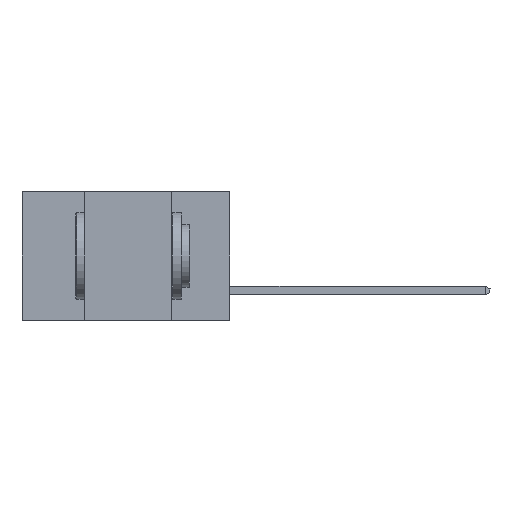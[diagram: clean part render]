
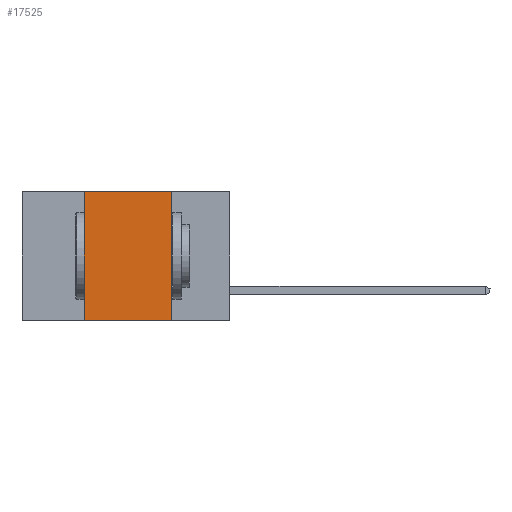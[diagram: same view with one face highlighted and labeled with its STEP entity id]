
A CAD part, left-side view. The second image highlights one B-rep face of the part: STEP entity #17525.
In plain terms, the highlighted planar face has unit normal (-1, 0, 0).
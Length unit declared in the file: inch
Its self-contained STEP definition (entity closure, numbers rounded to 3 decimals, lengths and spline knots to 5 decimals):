
#531 = AXIS2_PLACEMENT_3D ( 'NONE', #15701, #7742, #21314 ) ;
#1015 = EDGE_CURVE ( 'NONE', #6487, #20729, #23118, .T. ) ;
#1554 = CARTESIAN_POINT ( 'NONE',  ( 0., 0.17, -0.37 ) ) ;
#3136 = DIRECTION ( 'NONE',  ( 0., 0., -1. ) ) ;
#3268 = LINE ( 'NONE', #11237, #25562 ) ;
#4190 = LINE ( 'NONE', #19735, #8039 ) ;
#6487 = VERTEX_POINT ( 'NONE', #13993 ) ;
#6577 = EDGE_CURVE ( 'NONE', #20702, #20729, #4190, .T. ) ;
#6822 = EDGE_CURVE ( 'NONE', #20702, #9094, #3268, .T. ) ;
#7489 = FACE_OUTER_BOUND ( 'NONE', #17699, .T. ) ;
#7742 = DIRECTION ( 'NONE',  ( 1., 0., 0. ) ) ;
#8039 = VECTOR ( 'NONE', #10194, 39.37008 ) ;
#9094 = VERTEX_POINT ( 'NONE', #25158 ) ;
#10194 = DIRECTION ( 'NONE',  ( 0., -1., 0. ) ) ;
#11237 = CARTESIAN_POINT ( 'NONE',  ( 0., 0.42, -0.37 ) ) ;
#11472 = ORIENTED_EDGE ( 'NONE', *, *, #1015, .F. ) ;
#13035 = CARTESIAN_POINT ( 'NONE',  ( 0., 0.6, 0. ) ) ;
#13333 = PLANE ( 'NONE',  #531 ) ;
#13993 = CARTESIAN_POINT ( 'NONE',  ( 0., 0.17, 0. ) ) ;
#14577 = VECTOR ( 'NONE', #3136, 39.37008 ) ;
#14610 = ORIENTED_EDGE ( 'NONE', *, *, #6577, .T. ) ;
#15701 = CARTESIAN_POINT ( 'NONE',  ( 0., 0.6, 0. ) ) ;
#16845 = DIRECTION ( 'NONE',  ( 0., -1., 0. ) ) ;
#17107 = LINE ( 'NONE', #13035, #24840 ) ;
#17124 = DIRECTION ( 'NONE',  ( 0., 0., 1. ) ) ;
#17525 = ADVANCED_FACE ( 'NONE', ( #7489 ), #13333, .F. ) ;
#17699 = EDGE_LOOP ( 'NONE', ( #11472, #23010, #25480, #14610 ) ) ;
#19735 = CARTESIAN_POINT ( 'NONE',  ( 0., 0.6, -0.37 ) ) ;
#20020 = EDGE_CURVE ( 'NONE', #9094, #6487, #17107, .T. ) ;
#20427 = CARTESIAN_POINT ( 'NONE',  ( 0., 0.17, -0.37 ) ) ;
#20702 = VERTEX_POINT ( 'NONE', #23972 ) ;
#20729 = VERTEX_POINT ( 'NONE', #20427 ) ;
#21314 = DIRECTION ( 'NONE',  ( 0., 0., -1. ) ) ;
#23010 = ORIENTED_EDGE ( 'NONE', *, *, #20020, .F. ) ;
#23118 = LINE ( 'NONE', #1554, #14577 ) ;
#23972 = CARTESIAN_POINT ( 'NONE',  ( 0., 0.42, -0.37 ) ) ;
#24840 = VECTOR ( 'NONE', #16845, 39.37008 ) ;
#25158 = CARTESIAN_POINT ( 'NONE',  ( 0., 0.42, 0. ) ) ;
#25480 = ORIENTED_EDGE ( 'NONE', *, *, #6822, .F. ) ;
#25562 = VECTOR ( 'NONE', #17124, 39.37008 ) ;
